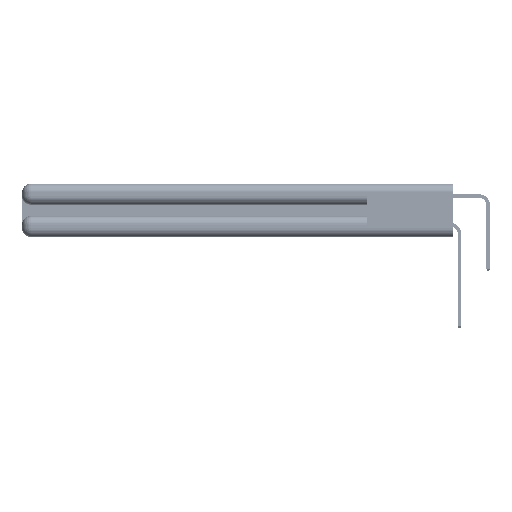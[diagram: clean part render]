
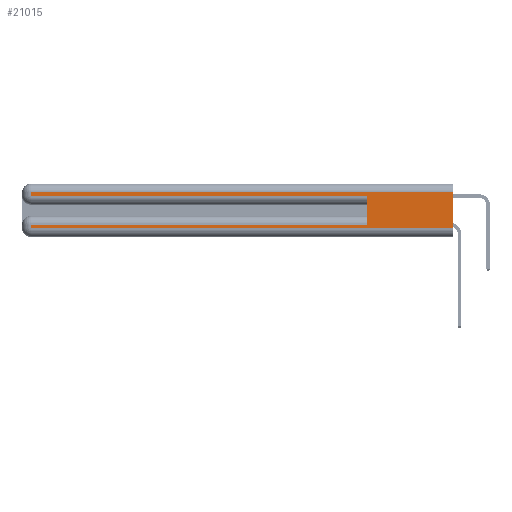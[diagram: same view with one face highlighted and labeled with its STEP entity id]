
A CAD part, left-side view. The second image highlights one B-rep face of the part: STEP entity #21015.
In plain terms, the highlighted planar face has unit normal (-1, 0, 0).
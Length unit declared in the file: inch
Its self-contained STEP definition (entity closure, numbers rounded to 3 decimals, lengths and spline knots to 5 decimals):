
#1236 = DIRECTION ( 'NONE',  ( 0., 0., -1. ) ) ;
#2004 = AXIS2_PLACEMENT_3D ( 'NONE', #41713, #46337, #19152 ) ;
#2581 = DIRECTION ( 'NONE',  ( 0., 1., 0. ) ) ;
#3660 = LINE ( 'NONE', #43347, #56670 ) ;
#4640 = VECTOR ( 'NONE', #34249, 39.37008 ) ;
#4986 = ORIENTED_EDGE ( 'NONE', *, *, #14005, .T. ) ;
#6367 = CARTESIAN_POINT ( 'NONE',  ( 0., 0., 0.285 ) ) ;
#8198 = VERTEX_POINT ( 'NONE', #51407 ) ;
#8347 = EDGE_CURVE ( 'NONE', #49981, #14325, #3660, .T. ) ;
#8742 = LINE ( 'NONE', #43651, #25864 ) ;
#8751 = VECTOR ( 'NONE', #41758, 39.37008 ) ;
#9781 = PLANE ( 'NONE',  #2004 ) ;
#9964 = EDGE_CURVE ( 'NONE', #51321, #57631, #51411, .T. ) ;
#11009 = VERTEX_POINT ( 'NONE', #34821 ) ;
#11504 = EDGE_CURVE ( 'NONE', #51321, #8198, #59097, .T. ) ;
#12299 = ORIENTED_EDGE ( 'NONE', *, *, #58843, .F. ) ;
#14005 = EDGE_CURVE ( 'NONE', #11009, #40688, #43656, .T. ) ;
#14061 = VECTOR ( 'NONE', #33552, 39.37008 ) ;
#14325 = VERTEX_POINT ( 'NONE', #22072 ) ;
#16272 = CARTESIAN_POINT ( 'NONE',  ( 0., 0., 0.31 ) ) ;
#17769 = ORIENTED_EDGE ( 'NONE', *, *, #11504, .T. ) ;
#19152 = DIRECTION ( 'NONE',  ( 0., 0., -1. ) ) ;
#19866 = VECTOR ( 'NONE', #1236, 39.37008 ) ;
#21015 = ADVANCED_FACE ( 'NONE', ( #46469 ), #9781, .F. ) ;
#21200 = CARTESIAN_POINT ( 'NONE',  ( 0., 0., 0.31 ) ) ;
#21493 = LINE ( 'NONE', #50611, #8751 ) ;
#22072 = CARTESIAN_POINT ( 'NONE',  ( 0., 2.94, 0.085 ) ) ;
#23911 = VECTOR ( 'NONE', #57481, 39.37008 ) ;
#25864 = VECTOR ( 'NONE', #53501, 39.37008 ) ;
#26948 = ORIENTED_EDGE ( 'NONE', *, *, #54339, .T. ) ;
#27308 = CARTESIAN_POINT ( 'NONE',  ( 0., 2.94, 0.06 ) ) ;
#28692 = CARTESIAN_POINT ( 'NONE',  ( 0., 0., 0.06 ) ) ;
#28957 = CARTESIAN_POINT ( 'NONE',  ( 0., 2.94, 0.37 ) ) ;
#31363 = ORIENTED_EDGE ( 'NONE', *, *, #58035, .T. ) ;
#32974 = ORIENTED_EDGE ( 'NONE', *, *, #8347, .T. ) ;
#33552 = DIRECTION ( 'NONE',  ( 0., 0., -1. ) ) ;
#34249 = DIRECTION ( 'NONE',  ( 0., -1., 0. ) ) ;
#34782 = CARTESIAN_POINT ( 'NONE',  ( 0., 0.6, 0.085 ) ) ;
#34821 = CARTESIAN_POINT ( 'NONE',  ( 0., 2.94, 0.285 ) ) ;
#38853 = CARTESIAN_POINT ( 'NONE',  ( 0., 0., 0.06 ) ) ;
#40496 = LINE ( 'NONE', #28957, #14061 ) ;
#40688 = VERTEX_POINT ( 'NONE', #44853 ) ;
#41713 = CARTESIAN_POINT ( 'NONE',  ( 0., 0., 0.37 ) ) ;
#41758 = DIRECTION ( 'NONE',  ( 0., 0., 1. ) ) ;
#41766 = CARTESIAN_POINT ( 'NONE',  ( 0., 0., 0.37 ) ) ;
#43347 = CARTESIAN_POINT ( 'NONE',  ( 0., 0., 0.085 ) ) ;
#43651 = CARTESIAN_POINT ( 'NONE',  ( 0., 2.94, 0.37 ) ) ;
#43656 = LINE ( 'NONE', #6367, #54469 ) ;
#43686 = DIRECTION ( 'NONE',  ( 0., -1., 0. ) ) ;
#44853 = CARTESIAN_POINT ( 'NONE',  ( 0., 0.6, 0.285 ) ) ;
#45438 = ORIENTED_EDGE ( 'NONE', *, *, #52470, .T. ) ;
#46337 = DIRECTION ( 'NONE',  ( 1., 0., 0. ) ) ;
#46469 = FACE_OUTER_BOUND ( 'NONE', #56809, .T. ) ;
#49551 = VERTEX_POINT ( 'NONE', #27308 ) ;
#49660 = LINE ( 'NONE', #38853, #4640 ) ;
#49981 = VERTEX_POINT ( 'NONE', #34782 ) ;
#50453 = ORIENTED_EDGE ( 'NONE', *, *, #9964, .F. ) ;
#50611 = CARTESIAN_POINT ( 'NONE',  ( 0., 0.6, 0.145 ) ) ;
#51321 = VERTEX_POINT ( 'NONE', #16272 ) ;
#51407 = CARTESIAN_POINT ( 'NONE',  ( 0., 2.94, 0.31 ) ) ;
#51411 = LINE ( 'NONE', #41766, #19866 ) ;
#52470 = EDGE_CURVE ( 'NONE', #8198, #11009, #40496, .T. ) ;
#53501 = DIRECTION ( 'NONE',  ( 0., 0., -1. ) ) ;
#54339 = EDGE_CURVE ( 'NONE', #49551, #57631, #49660, .T. ) ;
#54469 = VECTOR ( 'NONE', #43686, 39.37008 ) ;
#56670 = VECTOR ( 'NONE', #2581, 39.37008 ) ;
#56809 = EDGE_LOOP ( 'NONE', ( #50453, #17769, #45438, #4986, #12299, #32974, #31363, #26948 ) ) ;
#57481 = DIRECTION ( 'NONE',  ( 0., 1., 0. ) ) ;
#57631 = VERTEX_POINT ( 'NONE', #28692 ) ;
#58035 = EDGE_CURVE ( 'NONE', #14325, #49551, #8742, .T. ) ;
#58843 = EDGE_CURVE ( 'NONE', #49981, #40688, #21493, .T. ) ;
#59097 = LINE ( 'NONE', #21200, #23911 ) ;
